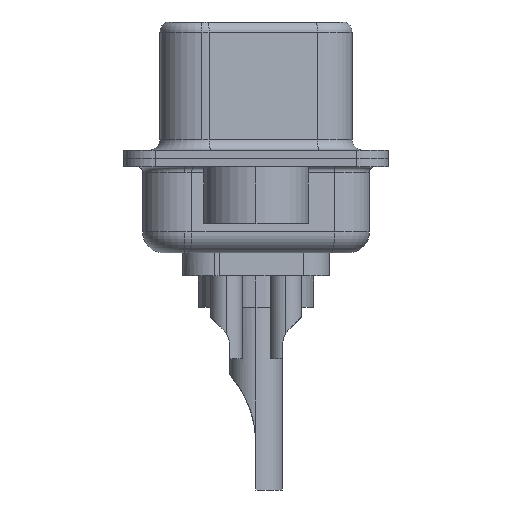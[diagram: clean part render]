
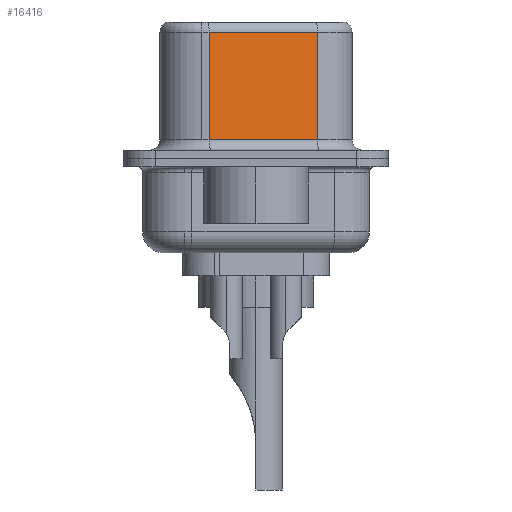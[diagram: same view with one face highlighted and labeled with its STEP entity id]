
A CAD part, left-side view. The second image highlights one B-rep face of the part: STEP entity #16416.
In plain terms, the highlighted planar face has unit normal (-0.985, -0.174, 0).
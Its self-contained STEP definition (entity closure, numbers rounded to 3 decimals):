
#989 = LINE ( 'NONE', #1546, #17115 ) ;
#1074 = LINE ( 'NONE', #16407, #17192 ) ;
#1280 = VERTEX_POINT ( 'NONE', #16468 ) ;
#1493 = AXIS2_PLACEMENT_3D ( 'NONE', #3521, #13049, #3582 ) ;
#1546 = CARTESIAN_POINT ( 'NONE',  ( 4.565, -2.927, 0.9 ) ) ;
#2008 = VECTOR ( 'NONE', #6192, 1000. ) ;
#2076 = CARTESIAN_POINT ( 'NONE',  ( 4.565, -2.927, 0.9 ) ) ;
#2615 = FACE_OUTER_BOUND ( 'NONE', #6771, .T. ) ;
#3521 = CARTESIAN_POINT ( 'NONE',  ( 4.565, -2.927, 6.52 ) ) ;
#3582 = DIRECTION ( 'NONE',  ( -0.174, 0.985, 0. ) ) ;
#4393 = ORIENTED_EDGE ( 'NONE', *, *, #4831, .T. ) ;
#4831 = EDGE_CURVE ( 'NONE', #17168, #5527, #1074, .T. ) ;
#5059 = VECTOR ( 'NONE', #11739, 1000. ) ;
#5527 = VERTEX_POINT ( 'NONE', #19737 ) ;
#6192 = DIRECTION ( 'NONE',  ( 0., 0., -1. ) ) ;
#6314 = LINE ( 'NONE', #12487, #2008 ) ;
#6771 = EDGE_LOOP ( 'NONE', ( #8375, #4393, #8196, #8063 ) ) ;
#8063 = ORIENTED_EDGE ( 'NONE', *, *, #19210, .T. ) ;
#8196 = ORIENTED_EDGE ( 'NONE', *, *, #18708, .T. ) ;
#8375 = ORIENTED_EDGE ( 'NONE', *, *, #19056, .F. ) ;
#8392 = DIRECTION ( 'NONE',  ( -0.174, 0.985, 0. ) ) ;
#9616 = CARTESIAN_POINT ( 'NONE',  ( 4.565, -2.927, 6.02 ) ) ;
#11739 = DIRECTION ( 'NONE',  ( 0., 0., -1. ) ) ;
#11757 = VERTEX_POINT ( 'NONE', #2076 ) ;
#12487 = CARTESIAN_POINT ( 'NONE',  ( 4.565, -2.927, 6.52 ) ) ;
#13049 = DIRECTION ( 'NONE',  ( 0.985, 0.174, 0. ) ) ;
#13246 = CARTESIAN_POINT ( 'NONE',  ( 3.655, 2.233, 6.52 ) ) ;
#13409 = LINE ( 'NONE', #13246, #5059 ) ;
#16407 = CARTESIAN_POINT ( 'NONE',  ( 4.565, -2.927, 6.02 ) ) ;
#16416 = ADVANCED_FACE ( 'NONE', ( #2615 ), #18990, .F. ) ;
#16468 = CARTESIAN_POINT ( 'NONE',  ( 3.655, 2.233, 0.9 ) ) ;
#17115 = VECTOR ( 'NONE', #20086, 1000. ) ;
#17168 = VERTEX_POINT ( 'NONE', #9616 ) ;
#17192 = VECTOR ( 'NONE', #8392, 1000. ) ;
#18708 = EDGE_CURVE ( 'NONE', #5527, #1280, #13409, .T. ) ;
#18990 = PLANE ( 'NONE',  #1493 ) ;
#19056 = EDGE_CURVE ( 'NONE', #17168, #11757, #6314, .T. ) ;
#19210 = EDGE_CURVE ( 'NONE', #1280, #11757, #989, .T. ) ;
#19737 = CARTESIAN_POINT ( 'NONE',  ( 3.655, 2.233, 6.02 ) ) ;
#20086 = DIRECTION ( 'NONE',  ( 0.174, -0.985, 0. ) ) ;
